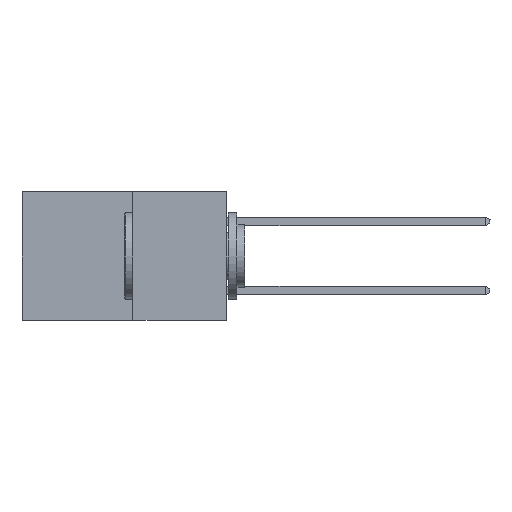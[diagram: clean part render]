
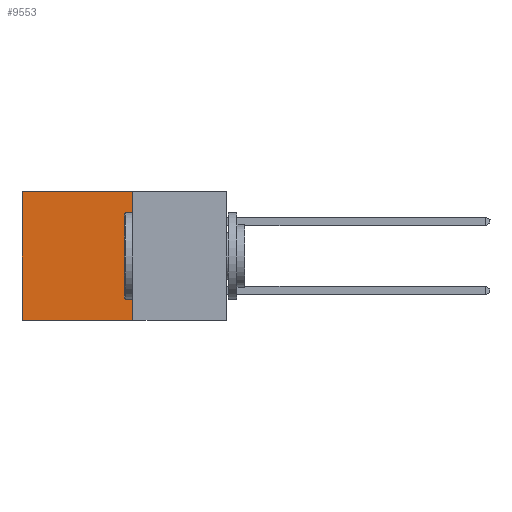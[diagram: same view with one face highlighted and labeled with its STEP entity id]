
A CAD part, left-side view. The second image highlights one B-rep face of the part: STEP entity #9553.
In plain terms, the highlighted planar face has unit normal (-1, 0, 0).
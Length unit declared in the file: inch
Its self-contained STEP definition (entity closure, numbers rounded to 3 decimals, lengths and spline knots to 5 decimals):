
#706 = PLANE ( 'NONE',  #2965 ) ;
#889 = DIRECTION ( 'NONE',  ( 0., 0., -1. ) ) ;
#922 = CARTESIAN_POINT ( 'NONE',  ( 0.277, 0.59, -0.37 ) ) ;
#1340 = LINE ( 'NONE', #13951, #24180 ) ;
#1521 = VECTOR ( 'NONE', #889, 39.37008 ) ;
#2965 = AXIS2_PLACEMENT_3D ( 'NONE', #16649, #2995, #18969 ) ;
#2995 = DIRECTION ( 'NONE',  ( 1., 0., 0. ) ) ;
#4205 = VERTEX_POINT ( 'NONE', #19843 ) ;
#5649 = EDGE_CURVE ( 'NONE', #23898, #25178, #19739, .T. ) ;
#7809 = LINE ( 'NONE', #11993, #13869 ) ;
#8443 = CARTESIAN_POINT ( 'NONE',  ( 0.277, 0.27, 0. ) ) ;
#8708 = EDGE_LOOP ( 'NONE', ( #13229, #19776, #16566, #11896 ) ) ;
#9553 = ADVANCED_FACE ( 'NONE', ( #11920 ), #706, .F. ) ;
#10336 = LINE ( 'NONE', #8443, #21787 ) ;
#11849 = EDGE_CURVE ( 'NONE', #4205, #23898, #10336, .T. ) ;
#11896 = ORIENTED_EDGE ( 'NONE', *, *, #11849, .T. ) ;
#11920 = FACE_OUTER_BOUND ( 'NONE', #8708, .T. ) ;
#11993 = CARTESIAN_POINT ( 'NONE',  ( 0.277, 0.27, -0.37 ) ) ;
#12596 = CARTESIAN_POINT ( 'NONE',  ( 0.277, 0.59, 0. ) ) ;
#13004 = DIRECTION ( 'NONE',  ( 0., 1., 0. ) ) ;
#13229 = ORIENTED_EDGE ( 'NONE', *, *, #5649, .T. ) ;
#13308 = EDGE_CURVE ( 'NONE', #14305, #25178, #7809, .T. ) ;
#13869 = VECTOR ( 'NONE', #25670, 39.37008 ) ;
#13951 = CARTESIAN_POINT ( 'NONE',  ( 0.277, 0.27, -0.37 ) ) ;
#14305 = VERTEX_POINT ( 'NONE', #15647 ) ;
#15647 = CARTESIAN_POINT ( 'NONE',  ( 0.277, 0.27, -0.37 ) ) ;
#16566 = ORIENTED_EDGE ( 'NONE', *, *, #26542, .F. ) ;
#16649 = CARTESIAN_POINT ( 'NONE',  ( 0.277, 0.27, -0.37 ) ) ;
#18601 = DIRECTION ( 'NONE',  ( 0., 0., -1. ) ) ;
#18969 = DIRECTION ( 'NONE',  ( 0., 0., -1. ) ) ;
#19739 = LINE ( 'NONE', #922, #1521 ) ;
#19776 = ORIENTED_EDGE ( 'NONE', *, *, #13308, .F. ) ;
#19843 = CARTESIAN_POINT ( 'NONE',  ( 0.277, 0.27, 0. ) ) ;
#21787 = VECTOR ( 'NONE', #13004, 39.37008 ) ;
#23740 = CARTESIAN_POINT ( 'NONE',  ( 0.277, 0.59, -0.37 ) ) ;
#23898 = VERTEX_POINT ( 'NONE', #12596 ) ;
#24180 = VECTOR ( 'NONE', #18601, 39.37008 ) ;
#25178 = VERTEX_POINT ( 'NONE', #23740 ) ;
#25670 = DIRECTION ( 'NONE',  ( 0., 1., 0. ) ) ;
#26542 = EDGE_CURVE ( 'NONE', #4205, #14305, #1340, .T. ) ;
